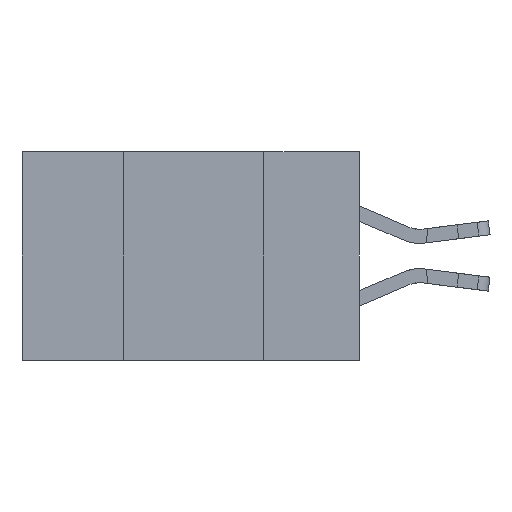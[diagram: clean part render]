
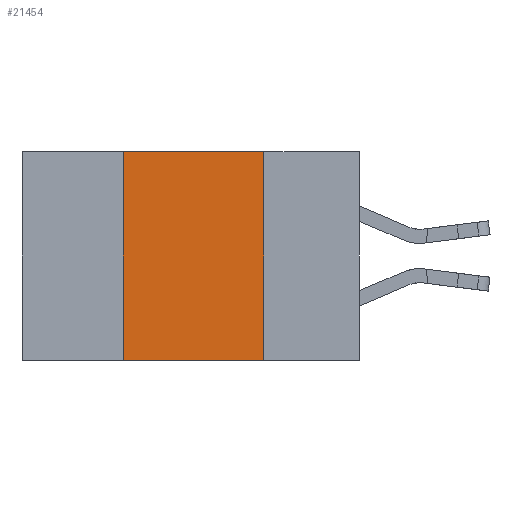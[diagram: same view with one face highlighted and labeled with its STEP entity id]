
A CAD part, left-side view. The second image highlights one B-rep face of the part: STEP entity #21454.
In plain terms, the highlighted planar face has unit normal (-1, 0, 0).
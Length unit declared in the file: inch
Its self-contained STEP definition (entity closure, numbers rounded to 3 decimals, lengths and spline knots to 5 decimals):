
#692 = DIRECTION ( 'NONE',  ( 0., -1., 0. ) ) ;
#1603 = VERTEX_POINT ( 'NONE', #7441 ) ;
#3903 = ORIENTED_EDGE ( 'NONE', *, *, #16866, .F. ) ;
#5413 = EDGE_LOOP ( 'NONE', ( #18684, #3903, #5784, #18544 ) ) ;
#5784 = ORIENTED_EDGE ( 'NONE', *, *, #17015, .F. ) ;
#6249 = VERTEX_POINT ( 'NONE', #19434 ) ;
#6273 = AXIS2_PLACEMENT_3D ( 'NONE', #12758, #19389, #17308 ) ;
#6802 = VECTOR ( 'NONE', #11466, 39.37008 ) ;
#6999 = EDGE_CURVE ( 'NONE', #6249, #11318, #7340, .T. ) ;
#7005 = CARTESIAN_POINT ( 'NONE',  ( 0., 0.42, -0.37 ) ) ;
#7201 = LINE ( 'NONE', #8727, #20798 ) ;
#7340 = LINE ( 'NONE', #19064, #15781 ) ;
#7441 = CARTESIAN_POINT ( 'NONE',  ( 0., 0.42, 0. ) ) ;
#8727 = CARTESIAN_POINT ( 'NONE',  ( 0., 0.6, -0.37 ) ) ;
#9289 = PLANE ( 'NONE',  #6273 ) ;
#10637 = CARTESIAN_POINT ( 'NONE',  ( 0., 0.6, 0. ) ) ;
#10645 = EDGE_CURVE ( 'NONE', #17089, #11318, #7201, .T. ) ;
#11247 = CARTESIAN_POINT ( 'NONE',  ( 0., 0.42, 0. ) ) ;
#11318 = VERTEX_POINT ( 'NONE', #11808 ) ;
#11466 = DIRECTION ( 'NONE',  ( 0., 0., 1. ) ) ;
#11808 = CARTESIAN_POINT ( 'NONE',  ( 0., 0.17, -0.37 ) ) ;
#12758 = CARTESIAN_POINT ( 'NONE',  ( 0., 0.6, 0. ) ) ;
#13830 = DIRECTION ( 'NONE',  ( 0., -1., 0. ) ) ;
#14089 = LINE ( 'NONE', #10637, #14424 ) ;
#14424 = VECTOR ( 'NONE', #692, 39.37008 ) ;
#15781 = VECTOR ( 'NONE', #16983, 39.37008 ) ;
#16115 = LINE ( 'NONE', #11247, #6802 ) ;
#16866 = EDGE_CURVE ( 'NONE', #1603, #6249, #14089, .T. ) ;
#16983 = DIRECTION ( 'NONE',  ( 0., 0., -1. ) ) ;
#17015 = EDGE_CURVE ( 'NONE', #17089, #1603, #16115, .T. ) ;
#17089 = VERTEX_POINT ( 'NONE', #7005 ) ;
#17308 = DIRECTION ( 'NONE',  ( 0., 0., -1. ) ) ;
#18544 = ORIENTED_EDGE ( 'NONE', *, *, #10645, .T. ) ;
#18684 = ORIENTED_EDGE ( 'NONE', *, *, #6999, .F. ) ;
#19064 = CARTESIAN_POINT ( 'NONE',  ( 0., 0.17, 0. ) ) ;
#19290 = FACE_OUTER_BOUND ( 'NONE', #5413, .T. ) ;
#19389 = DIRECTION ( 'NONE',  ( 1., 0., 0. ) ) ;
#19434 = CARTESIAN_POINT ( 'NONE',  ( 0., 0.17, 0. ) ) ;
#20798 = VECTOR ( 'NONE', #13830, 39.37008 ) ;
#21454 = ADVANCED_FACE ( 'NONE', ( #19290 ), #9289, .F. ) ;
